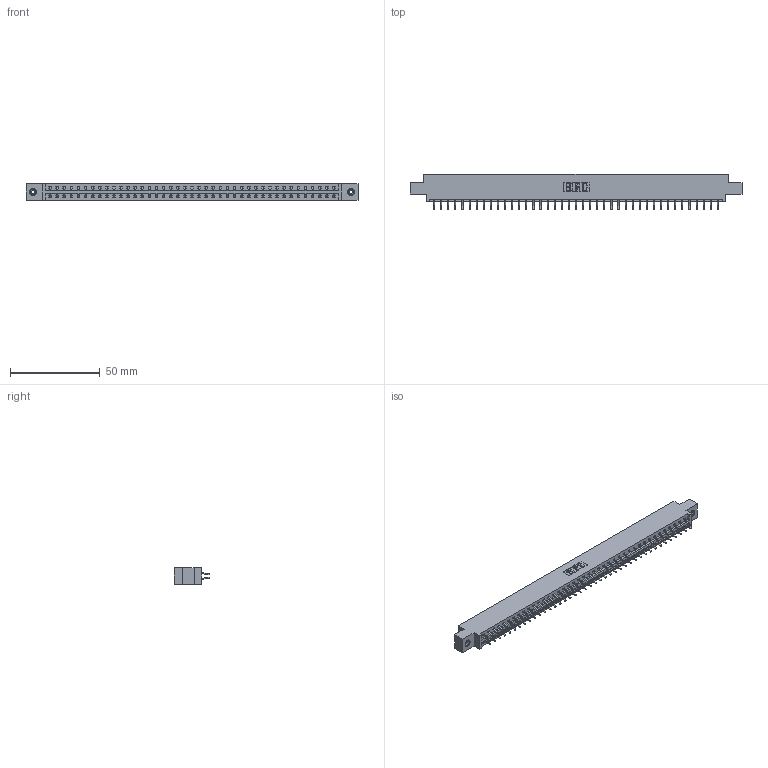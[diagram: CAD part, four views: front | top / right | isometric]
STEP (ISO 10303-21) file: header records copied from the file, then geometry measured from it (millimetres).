
FILE_DESCRIPTION (( 'STEP AP203' ), '1' );
FILE_NAME ('337-082-556-808.STEP', '2018-08-12T21:04:06', ( '' ), ( '' ), 'SwSTEP 2.0', 'SolidWorks 2016', '' );
FILE_SCHEMA (( 'CONFIG_CONTROL_DESIGN' ));
Length unit declared in the file: inch
Products named in the file (4): 345-250-001_345-250-003-102; 337-082-556-808; 345-292-001_556 Tail; 337 Part_0.170 Offset - 0.156 Dia-TI
Assembly tree (85 placements, depth 2):
  337-082-556-808
    337 Part_0.170 Offset - 0.156 Dia-TI
    345-292-001_556 Tail  x82
    345-250-001_345-250-003-102  x2
Bounding box: 185.47 x 19.57 x 9.4 mm (x, y, z)
Volume: 19405.8 mm3; surface area: 21973.8 mm2
Topology: 85 solids, 85 shells, 5098 faces, 15137 edges, 9974 vertices
Faces by surface type: plane 3550, cylinder 1532, cone 12, torus 4
Entity records: 33456 total; most frequent: CARTESIAN_POINT 5633, ORIENTED_EDGE 5550, DIRECTION 4813, EDGE_CURVE 2775, LINE 2619, VECTOR 2619, VERTEX_POINT 1844, AXIS2_PLACEMENT_3D 1097
